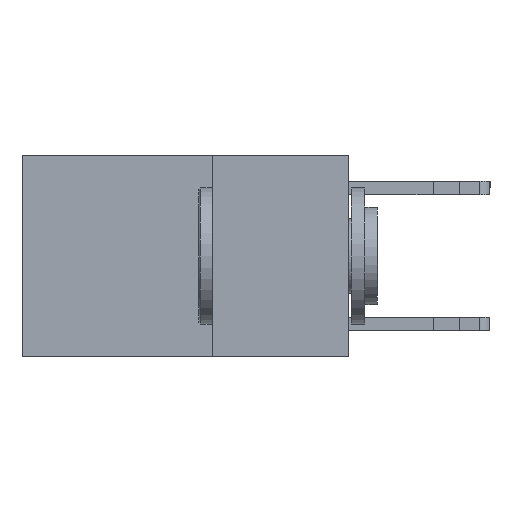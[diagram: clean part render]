
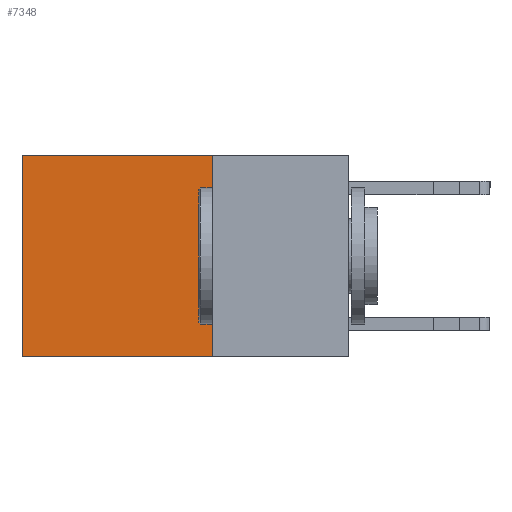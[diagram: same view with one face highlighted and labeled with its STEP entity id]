
A CAD part, left-side view. The second image highlights one B-rep face of the part: STEP entity #7348.
In plain terms, the highlighted planar face has unit normal (-1, 0, 0).
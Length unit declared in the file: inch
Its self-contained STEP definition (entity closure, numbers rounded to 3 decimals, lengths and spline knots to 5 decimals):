
#1244 = EDGE_LOOP ( 'NONE', ( #20878, #8079, #18697, #6216 ) ) ;
#1825 = DIRECTION ( 'NONE',  ( 0., 0., -1. ) ) ;
#1995 = AXIS2_PLACEMENT_3D ( 'NONE', #9045, #15682, #18933 ) ;
#2680 = CARTESIAN_POINT ( 'NONE',  ( 0.2625, 0.25, 0. ) ) ;
#3671 = LINE ( 'NONE', #8618, #9388 ) ;
#4545 = VERTEX_POINT ( 'NONE', #16620 ) ;
#5289 = DIRECTION ( 'NONE',  ( 0., 0., -1. ) ) ;
#5389 = CARTESIAN_POINT ( 'NONE',  ( 0.2625, 0.25, 0. ) ) ;
#5673 = VECTOR ( 'NONE', #16117, 39.37008 ) ;
#6216 = ORIENTED_EDGE ( 'NONE', *, *, #18625, .T. ) ;
#6885 = CARTESIAN_POINT ( 'NONE',  ( 0.2625, 0.25, -0.37 ) ) ;
#7323 = VERTEX_POINT ( 'NONE', #2680 ) ;
#7348 = ADVANCED_FACE ( 'NONE', ( #9459 ), #19141, .F. ) ;
#7588 = CARTESIAN_POINT ( 'NONE',  ( 0.2625, 0.6, -0.37 ) ) ;
#8079 = ORIENTED_EDGE ( 'NONE', *, *, #18767, .F. ) ;
#8618 = CARTESIAN_POINT ( 'NONE',  ( 0.2625, 0.6, 0. ) ) ;
#9026 = EDGE_CURVE ( 'NONE', #7323, #4545, #13416, .T. ) ;
#9045 = CARTESIAN_POINT ( 'NONE',  ( 0.2625, 0.25, 0. ) ) ;
#9388 = VECTOR ( 'NONE', #1825, 39.37008 ) ;
#9459 = FACE_OUTER_BOUND ( 'NONE', #1244, .T. ) ;
#12518 = VECTOR ( 'NONE', #13414, 39.37008 ) ;
#12551 = VERTEX_POINT ( 'NONE', #7588 ) ;
#13038 = VERTEX_POINT ( 'NONE', #20576 ) ;
#13414 = DIRECTION ( 'NONE',  ( 0., 1., 0. ) ) ;
#13416 = LINE ( 'NONE', #5389, #18682 ) ;
#15682 = DIRECTION ( 'NONE',  ( 1., 0., 0. ) ) ;
#16117 = DIRECTION ( 'NONE',  ( 0., 1., 0. ) ) ;
#16233 = CARTESIAN_POINT ( 'NONE',  ( 0.2625, 0.25, 0. ) ) ;
#16620 = CARTESIAN_POINT ( 'NONE',  ( 0.2625, 0.25, -0.37 ) ) ;
#16941 = EDGE_CURVE ( 'NONE', #13038, #12551, #3671, .T. ) ;
#18374 = LINE ( 'NONE', #6885, #12518 ) ;
#18625 = EDGE_CURVE ( 'NONE', #7323, #13038, #19576, .T. ) ;
#18682 = VECTOR ( 'NONE', #5289, 39.37008 ) ;
#18697 = ORIENTED_EDGE ( 'NONE', *, *, #9026, .F. ) ;
#18767 = EDGE_CURVE ( 'NONE', #4545, #12551, #18374, .T. ) ;
#18933 = DIRECTION ( 'NONE',  ( 0., 0., -1. ) ) ;
#19141 = PLANE ( 'NONE',  #1995 ) ;
#19576 = LINE ( 'NONE', #16233, #5673 ) ;
#20576 = CARTESIAN_POINT ( 'NONE',  ( 0.2625, 0.6, 0. ) ) ;
#20878 = ORIENTED_EDGE ( 'NONE', *, *, #16941, .T. ) ;
